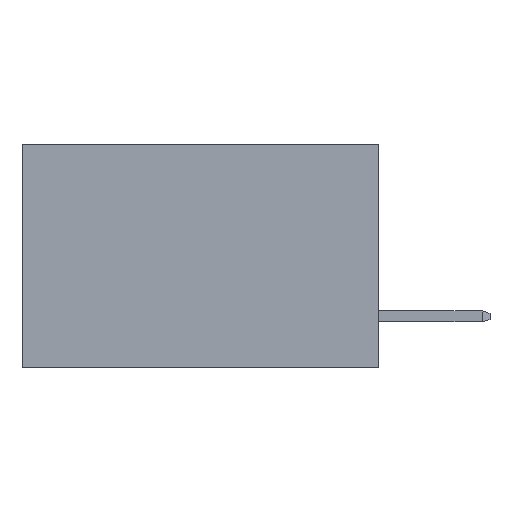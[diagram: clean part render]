
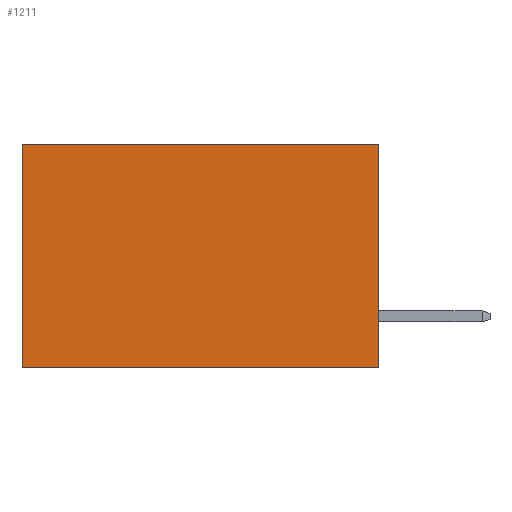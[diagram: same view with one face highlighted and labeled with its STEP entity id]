
A CAD part, left-side view. The second image highlights one B-rep face of the part: STEP entity #1211.
In plain terms, the highlighted planar face has unit normal (-1, 0, 0).
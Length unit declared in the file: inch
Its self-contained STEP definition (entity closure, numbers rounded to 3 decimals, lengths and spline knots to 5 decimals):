
#61 = CARTESIAN_POINT ( 'NONE',  ( 0.277, 0.59, -0.37 ) ) ;
#97 = CARTESIAN_POINT ( 'NONE',  ( 0.277, 0., 0. ) ) ;
#314 = CARTESIAN_POINT ( 'NONE',  ( 0.277, 0.59, -0.37 ) ) ;
#1109 = DIRECTION ( 'NONE',  ( 0., 0., -1. ) ) ;
#1211 = ADVANCED_FACE ( 'NONE', ( #1584 ), #7527, .F. ) ;
#1220 = LINE ( 'NONE', #3652, #6373 ) ;
#1366 = DIRECTION ( 'NONE',  ( 0., 0., -1. ) ) ;
#1384 = ORIENTED_EDGE ( 'NONE', *, *, #8134, .T. ) ;
#1584 = FACE_OUTER_BOUND ( 'NONE', #3207, .T. ) ;
#1763 = VERTEX_POINT ( 'NONE', #61 ) ;
#2238 = AXIS2_PLACEMENT_3D ( 'NONE', #6818, #7692, #1366 ) ;
#3207 = EDGE_LOOP ( 'NONE', ( #5864, #7116, #5503, #1384 ) ) ;
#3535 = LINE ( 'NONE', #314, #6948 ) ;
#3555 = LINE ( 'NONE', #97, #6969 ) ;
#3652 = CARTESIAN_POINT ( 'NONE',  ( 0.277, 0., -0.37 ) ) ;
#3720 = CARTESIAN_POINT ( 'NONE',  ( 0.277, 0.59, 0. ) ) ;
#3759 = DIRECTION ( 'NONE',  ( 0., 1., 0. ) ) ;
#4345 = DIRECTION ( 'NONE',  ( 0., 1., 0. ) ) ;
#4386 = CARTESIAN_POINT ( 'NONE',  ( 0.277, 0., 0. ) ) ;
#4525 = VERTEX_POINT ( 'NONE', #4386 ) ;
#4792 = LINE ( 'NONE', #5051, #8138 ) ;
#5039 = DIRECTION ( 'NONE',  ( 0., 0., -1. ) ) ;
#5051 = CARTESIAN_POINT ( 'NONE',  ( 0.277, 0., -0.37 ) ) ;
#5306 = VERTEX_POINT ( 'NONE', #6499 ) ;
#5503 = ORIENTED_EDGE ( 'NONE', *, *, #5613, .F. ) ;
#5613 = EDGE_CURVE ( 'NONE', #4525, #5306, #4792, .T. ) ;
#5864 = ORIENTED_EDGE ( 'NONE', *, *, #8878, .T. ) ;
#6373 = VECTOR ( 'NONE', #4345, 39.37008 ) ;
#6499 = CARTESIAN_POINT ( 'NONE',  ( 0.277, 0., -0.37 ) ) ;
#6734 = VERTEX_POINT ( 'NONE', #3720 ) ;
#6818 = CARTESIAN_POINT ( 'NONE',  ( 0.277, 0., -0.37 ) ) ;
#6948 = VECTOR ( 'NONE', #1109, 39.37008 ) ;
#6969 = VECTOR ( 'NONE', #3759, 39.37008 ) ;
#7116 = ORIENTED_EDGE ( 'NONE', *, *, #7264, .F. ) ;
#7264 = EDGE_CURVE ( 'NONE', #5306, #1763, #1220, .T. ) ;
#7527 = PLANE ( 'NONE',  #2238 ) ;
#7692 = DIRECTION ( 'NONE',  ( 1., 0., 0. ) ) ;
#8134 = EDGE_CURVE ( 'NONE', #4525, #6734, #3555, .T. ) ;
#8138 = VECTOR ( 'NONE', #5039, 39.37008 ) ;
#8878 = EDGE_CURVE ( 'NONE', #6734, #1763, #3535, .T. ) ;
